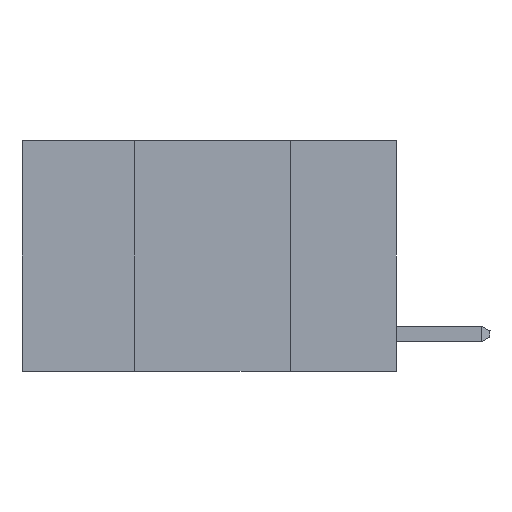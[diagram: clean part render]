
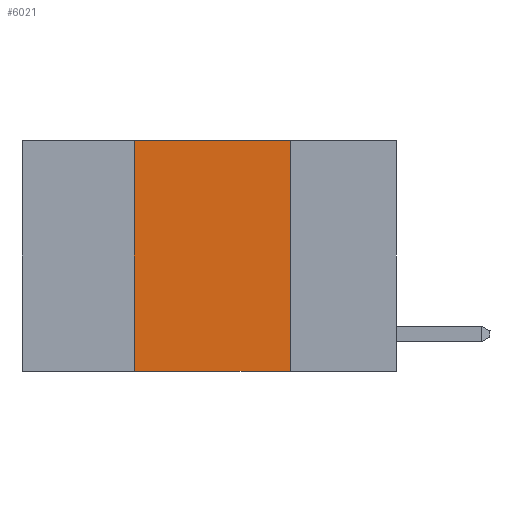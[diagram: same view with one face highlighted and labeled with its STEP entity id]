
A CAD part, left-side view. The second image highlights one B-rep face of the part: STEP entity #6021.
In plain terms, the highlighted planar face has unit normal (-1, 0, 0).
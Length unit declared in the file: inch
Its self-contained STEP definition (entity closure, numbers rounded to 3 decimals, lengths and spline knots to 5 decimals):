
#1054 = ORIENTED_EDGE ( 'NONE', *, *, #12893, .T. ) ;
#1647 = DIRECTION ( 'NONE',  ( 0., 0., -1. ) ) ;
#1799 = CARTESIAN_POINT ( 'NONE',  ( 0., 0.17, 0. ) ) ;
#3060 = VERTEX_POINT ( 'NONE', #3876 ) ;
#3509 = ORIENTED_EDGE ( 'NONE', *, *, #9054, .F. ) ;
#3784 = VECTOR ( 'NONE', #1647, 39.37008 ) ;
#3876 = CARTESIAN_POINT ( 'NONE',  ( 0., 0.42, 0. ) ) ;
#4191 = CARTESIAN_POINT ( 'NONE',  ( 0., 0.6, 0. ) ) ;
#4274 = FACE_OUTER_BOUND ( 'NONE', #10385, .T. ) ;
#5152 = CARTESIAN_POINT ( 'NONE',  ( 0., 0.6, 0. ) ) ;
#5228 = DIRECTION ( 'NONE',  ( 0., -1., 0. ) ) ;
#5580 = CARTESIAN_POINT ( 'NONE',  ( 0., 0.6, -0.37 ) ) ;
#5734 = CARTESIAN_POINT ( 'NONE',  ( 0., 0.42, -0.37 ) ) ;
#5812 = DIRECTION ( 'NONE',  ( 0., -1., 0. ) ) ;
#5898 = VECTOR ( 'NONE', #16313, 39.37008 ) ;
#6021 = ADVANCED_FACE ( 'NONE', ( #4274 ), #7766, .F. ) ;
#6170 = ORIENTED_EDGE ( 'NONE', *, *, #11759, .F. ) ;
#6517 = DIRECTION ( 'NONE',  ( 0., 0., -1. ) ) ;
#7766 = PLANE ( 'NONE',  #13516 ) ;
#7775 = LINE ( 'NONE', #15225, #5898 ) ;
#8460 = LINE ( 'NONE', #5580, #11389 ) ;
#9054 = EDGE_CURVE ( 'NONE', #12360, #16408, #9426, .T. ) ;
#9426 = LINE ( 'NONE', #1799, #3784 ) ;
#9433 = VERTEX_POINT ( 'NONE', #5734 ) ;
#9757 = VECTOR ( 'NONE', #5228, 39.37008 ) ;
#10316 = CARTESIAN_POINT ( 'NONE',  ( 0., 0.17, -0.37 ) ) ;
#10385 = EDGE_LOOP ( 'NONE', ( #3509, #14631, #6170, #1054 ) ) ;
#10579 = CARTESIAN_POINT ( 'NONE',  ( 0., 0.17, 0. ) ) ;
#11389 = VECTOR ( 'NONE', #5812, 39.37008 ) ;
#11759 = EDGE_CURVE ( 'NONE', #9433, #3060, #7775, .T. ) ;
#12360 = VERTEX_POINT ( 'NONE', #10579 ) ;
#12870 = DIRECTION ( 'NONE',  ( 1., 0., 0. ) ) ;
#12893 = EDGE_CURVE ( 'NONE', #9433, #16408, #8460, .T. ) ;
#13233 = EDGE_CURVE ( 'NONE', #3060, #12360, #14142, .T. ) ;
#13516 = AXIS2_PLACEMENT_3D ( 'NONE', #4191, #12870, #6517 ) ;
#14142 = LINE ( 'NONE', #5152, #9757 ) ;
#14631 = ORIENTED_EDGE ( 'NONE', *, *, #13233, .F. ) ;
#15225 = CARTESIAN_POINT ( 'NONE',  ( 0., 0.42, 0. ) ) ;
#16313 = DIRECTION ( 'NONE',  ( 0., 0., 1. ) ) ;
#16408 = VERTEX_POINT ( 'NONE', #10316 ) ;
